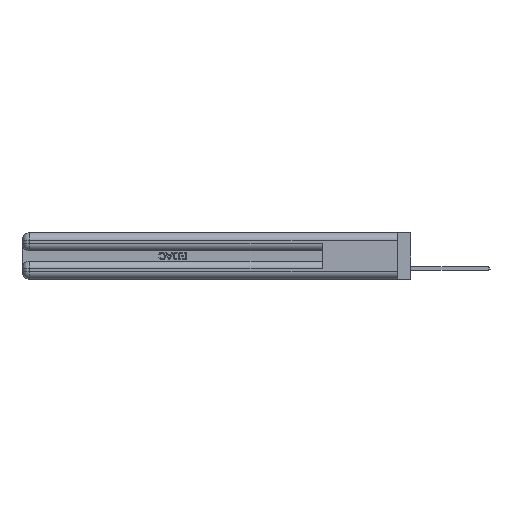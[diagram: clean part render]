
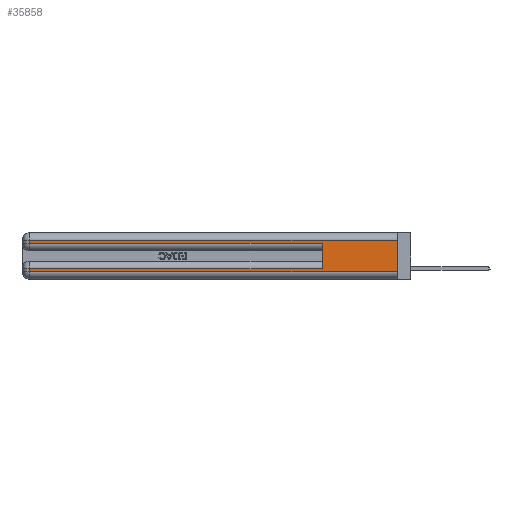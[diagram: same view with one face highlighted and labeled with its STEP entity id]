
A CAD part, left-side view. The second image highlights one B-rep face of the part: STEP entity #35858.
In plain terms, the highlighted planar face has unit normal (-1, 0, 0).
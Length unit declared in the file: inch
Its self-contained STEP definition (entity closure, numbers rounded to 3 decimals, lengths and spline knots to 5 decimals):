
#60 = ORIENTED_EDGE ( 'NONE', *, *, #13812, .T. ) ;
#1432 = DIRECTION ( 'NONE',  ( 0., -1., 0. ) ) ;
#1470 = CARTESIAN_POINT ( 'NONE',  ( 0., 2.94, 0.285 ) ) ;
#1955 = EDGE_CURVE ( 'NONE', #41997, #6482, #3786, .T. ) ;
#2222 = CARTESIAN_POINT ( 'NONE',  ( 0., 0., 0.37 ) ) ;
#2675 = LINE ( 'NONE', #45982, #28442 ) ;
#3370 = CARTESIAN_POINT ( 'NONE',  ( 0., 2.94, 0.085 ) ) ;
#3509 = ORIENTED_EDGE ( 'NONE', *, *, #1955, .F. ) ;
#3773 = EDGE_CURVE ( 'NONE', #41997, #14994, #41897, .T. ) ;
#3786 = LINE ( 'NONE', #22543, #11230 ) ;
#4632 = DIRECTION ( 'NONE',  ( 0., 0., 1. ) ) ;
#5145 = CARTESIAN_POINT ( 'NONE',  ( 0., 0.6, 0.285 ) ) ;
#5993 = EDGE_CURVE ( 'NONE', #45936, #33353, #2675, .T. ) ;
#6461 = EDGE_CURVE ( 'NONE', #17131, #6482, #16332, .T. ) ;
#6482 = VERTEX_POINT ( 'NONE', #5145 ) ;
#8816 = CARTESIAN_POINT ( 'NONE',  ( 0., 0., 0.31 ) ) ;
#9581 = EDGE_CURVE ( 'NONE', #38055, #17131, #37445, .T. ) ;
#10202 = DIRECTION ( 'NONE',  ( 0., -1., 0. ) ) ;
#10778 = EDGE_CURVE ( 'NONE', #18624, #33353, #46549, .T. ) ;
#11139 = CARTESIAN_POINT ( 'NONE',  ( 0., 0., 0.31 ) ) ;
#11230 = VECTOR ( 'NONE', #4632, 39.37008 ) ;
#13812 = EDGE_CURVE ( 'NONE', #45936, #38055, #41933, .T. ) ;
#14715 = ORIENTED_EDGE ( 'NONE', *, *, #9581, .T. ) ;
#14994 = VERTEX_POINT ( 'NONE', #3370 ) ;
#15281 = ORIENTED_EDGE ( 'NONE', *, *, #5993, .F. ) ;
#16149 = EDGE_LOOP ( 'NONE', ( #15281, #60, #14715, #30207, #3509, #37659, #30683, #26913 ) ) ;
#16160 = VECTOR ( 'NONE', #17837, 39.37008 ) ;
#16332 = LINE ( 'NONE', #23850, #23198 ) ;
#16960 = VECTOR ( 'NONE', #38606, 39.37008 ) ;
#17115 = DIRECTION ( 'NONE',  ( 0., 0., -1. ) ) ;
#17131 = VERTEX_POINT ( 'NONE', #1470 ) ;
#17837 = DIRECTION ( 'NONE',  ( 0., 1., 0. ) ) ;
#18624 = VERTEX_POINT ( 'NONE', #46299 ) ;
#19521 = CARTESIAN_POINT ( 'NONE',  ( 0., 0.6, 0.085 ) ) ;
#19703 = AXIS2_PLACEMENT_3D ( 'NONE', #2222, #27829, #38845 ) ;
#20247 = CARTESIAN_POINT ( 'NONE',  ( 0., 2.94, 0.37 ) ) ;
#22024 = VECTOR ( 'NONE', #17115, 39.37008 ) ;
#22170 = DIRECTION ( 'NONE',  ( 0., 1., 0. ) ) ;
#22543 = CARTESIAN_POINT ( 'NONE',  ( 0., 0.6, 0.145 ) ) ;
#23198 = VECTOR ( 'NONE', #1432, 39.37008 ) ;
#23850 = CARTESIAN_POINT ( 'NONE',  ( 0., 0., 0.285 ) ) ;
#24070 = DIRECTION ( 'NONE',  ( 0., 0., -1. ) ) ;
#26913 = ORIENTED_EDGE ( 'NONE', *, *, #10778, .T. ) ;
#27048 = VECTOR ( 'NONE', #10202, 39.37008 ) ;
#27829 = DIRECTION ( 'NONE',  ( 1., 0., 0. ) ) ;
#28442 = VECTOR ( 'NONE', #24070, 39.37008 ) ;
#30207 = ORIENTED_EDGE ( 'NONE', *, *, #6461, .T. ) ;
#30683 = ORIENTED_EDGE ( 'NONE', *, *, #37910, .T. ) ;
#31642 = CARTESIAN_POINT ( 'NONE',  ( 0., 2.94, 0.37 ) ) ;
#33353 = VERTEX_POINT ( 'NONE', #41458 ) ;
#35858 = ADVANCED_FACE ( 'NONE', ( #43968 ), #46053, .F. ) ;
#36383 = LINE ( 'NONE', #20247, #16960 ) ;
#36521 = CARTESIAN_POINT ( 'NONE',  ( 0., 0., 0.085 ) ) ;
#37445 = LINE ( 'NONE', #31642, #22024 ) ;
#37659 = ORIENTED_EDGE ( 'NONE', *, *, #3773, .T. ) ;
#37910 = EDGE_CURVE ( 'NONE', #14994, #18624, #36383, .T. ) ;
#38055 = VERTEX_POINT ( 'NONE', #46644 ) ;
#38606 = DIRECTION ( 'NONE',  ( 0., 0., -1. ) ) ;
#38845 = DIRECTION ( 'NONE',  ( 0., 0., -1. ) ) ;
#41458 = CARTESIAN_POINT ( 'NONE',  ( 0., 0., 0.06 ) ) ;
#41897 = LINE ( 'NONE', #36521, #16160 ) ;
#41933 = LINE ( 'NONE', #11139, #45938 ) ;
#41997 = VERTEX_POINT ( 'NONE', #19521 ) ;
#43968 = FACE_OUTER_BOUND ( 'NONE', #16149, .T. ) ;
#45936 = VERTEX_POINT ( 'NONE', #8816 ) ;
#45938 = VECTOR ( 'NONE', #22170, 39.37008 ) ;
#45982 = CARTESIAN_POINT ( 'NONE',  ( 0., 0., 0.37 ) ) ;
#46053 = PLANE ( 'NONE',  #19703 ) ;
#46299 = CARTESIAN_POINT ( 'NONE',  ( 0., 2.94, 0.06 ) ) ;
#46549 = LINE ( 'NONE', #46834, #27048 ) ;
#46644 = CARTESIAN_POINT ( 'NONE',  ( 0., 2.94, 0.31 ) ) ;
#46834 = CARTESIAN_POINT ( 'NONE',  ( 0., 0., 0.06 ) ) ;
